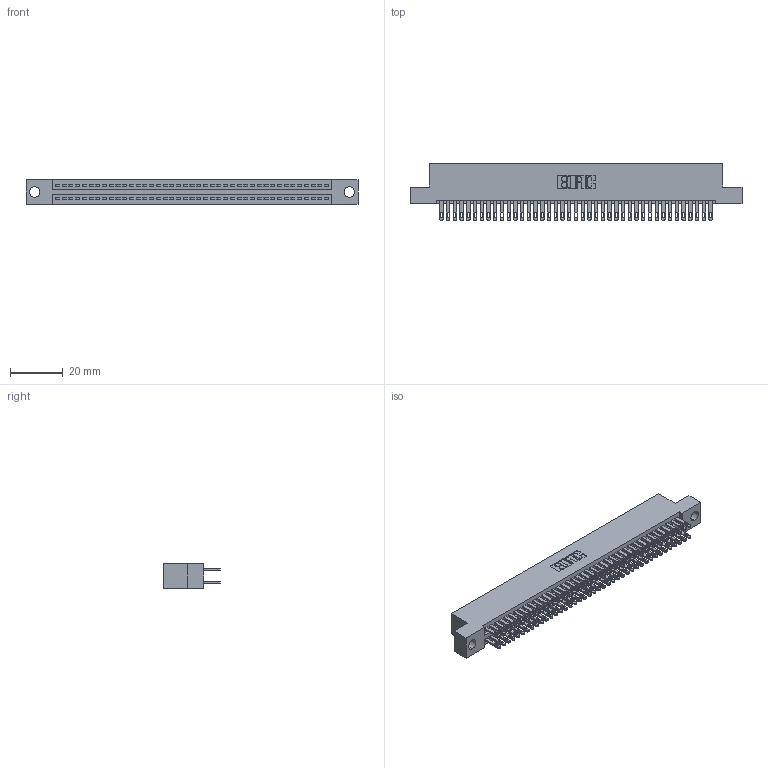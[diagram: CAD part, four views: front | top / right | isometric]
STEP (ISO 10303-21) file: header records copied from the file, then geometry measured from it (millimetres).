
FILE_DESCRIPTION (( 'STEP AP203' ), '1' );
FILE_NAME ('345-082-500-204.STEP', '2021-05-20T11:46:20', ( '' ), ( '' ), 'SwSTEP 2.0', 'SolidWorks 2020', '' );
FILE_SCHEMA (( 'CONFIG_CONTROL_DESIGN' ));
Length unit declared in the file: inch
Products named in the file (3): 345-292-001_345-293-100; 345 Part_Flush Mounting Lugs - 0.156 Dia-TI; 345-082-500-204
Assembly tree (83 placements, depth 2):
  345-082-500-204
    345 Part_Flush Mounting Lugs - 0.156 Dia-TI
    345-292-001_345-293-100  x82
Bounding box: 125.35 x 21.51 x 9.4 mm (x, y, z)
Volume: 12311.9 mm3; surface area: 18867.6 mm2
Topology: 83 solids, 83 shells, 3912 faces, 11939 edges, 7958 vertices
Faces by surface type: plane 2308, cylinder 1604
Entity records: 32653 total; most frequent: CARTESIAN_POINT 5478, ORIENTED_EDGE 5410, DIRECTION 4833, EDGE_CURVE 2705, LINE 2405, VECTOR 2405, VERTEX_POINT 1802, AXIS2_PLACEMENT_3D 1214
